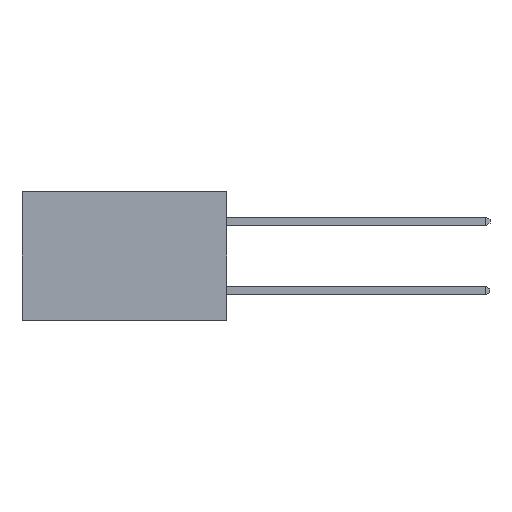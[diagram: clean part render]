
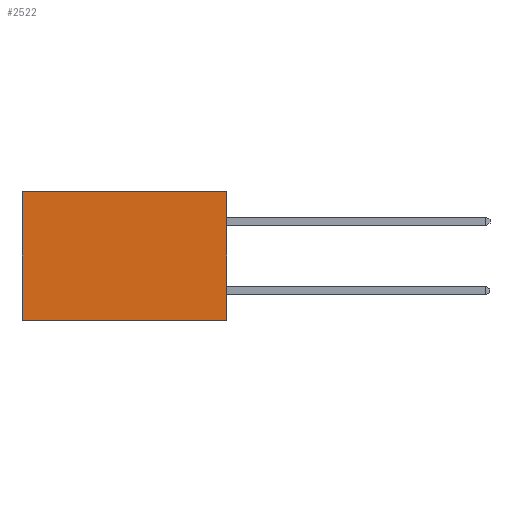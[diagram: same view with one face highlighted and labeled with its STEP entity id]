
A CAD part, left-side view. The second image highlights one B-rep face of the part: STEP entity #2522.
In plain terms, the highlighted planar face has unit normal (-1, 0, 0).
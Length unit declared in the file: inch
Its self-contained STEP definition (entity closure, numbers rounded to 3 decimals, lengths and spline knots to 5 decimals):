
#405 = ORIENTED_EDGE ( 'NONE', *, *, #4401, .F. ) ;
#432 = DIRECTION ( 'NONE',  ( 1., 0., 0. ) ) ;
#1007 = EDGE_LOOP ( 'NONE', ( #6013, #7449, #405, #2501 ) ) ;
#1068 = CARTESIAN_POINT ( 'NONE',  ( 0.277, 0., 0. ) ) ;
#1666 = PLANE ( 'NONE',  #2136 ) ;
#2136 = AXIS2_PLACEMENT_3D ( 'NONE', #5422, #432, #4265 ) ;
#2160 = CARTESIAN_POINT ( 'NONE',  ( 0.277, 0.59, 0. ) ) ;
#2501 = ORIENTED_EDGE ( 'NONE', *, *, #6601, .T. ) ;
#2522 = ADVANCED_FACE ( 'NONE', ( #6278 ), #1666, .F. ) ;
#2627 = CARTESIAN_POINT ( 'NONE',  ( 0.277, 0.59, -0.37 ) ) ;
#2742 = VERTEX_POINT ( 'NONE', #2160 ) ;
#2931 = VERTEX_POINT ( 'NONE', #2627 ) ;
#3594 = LINE ( 'NONE', #4609, #6913 ) ;
#3935 = LINE ( 'NONE', #6629, #7133 ) ;
#4180 = CARTESIAN_POINT ( 'NONE',  ( 0.277, 0., -0.37 ) ) ;
#4265 = DIRECTION ( 'NONE',  ( 0., 0., -1. ) ) ;
#4401 = EDGE_CURVE ( 'NONE', #7000, #7914, #8371, .T. ) ;
#4413 = EDGE_CURVE ( 'NONE', #7914, #2931, #5652, .T. ) ;
#4569 = DIRECTION ( 'NONE',  ( 0., 0., -1. ) ) ;
#4609 = CARTESIAN_POINT ( 'NONE',  ( 0.277, 0.59, -0.37 ) ) ;
#5014 = DIRECTION ( 'NONE',  ( 0., 0., -1. ) ) ;
#5415 = VECTOR ( 'NONE', #7773, 39.37008 ) ;
#5422 = CARTESIAN_POINT ( 'NONE',  ( 0.277, 0., -0.37 ) ) ;
#5652 = LINE ( 'NONE', #7811, #5415 ) ;
#6013 = ORIENTED_EDGE ( 'NONE', *, *, #6222, .T. ) ;
#6222 = EDGE_CURVE ( 'NONE', #2742, #2931, #3594, .T. ) ;
#6278 = FACE_OUTER_BOUND ( 'NONE', #1007, .T. ) ;
#6601 = EDGE_CURVE ( 'NONE', #7000, #2742, #3935, .T. ) ;
#6629 = CARTESIAN_POINT ( 'NONE',  ( 0.277, 0., 0. ) ) ;
#6913 = VECTOR ( 'NONE', #4569, 39.37008 ) ;
#7000 = VERTEX_POINT ( 'NONE', #1068 ) ;
#7029 = VECTOR ( 'NONE', #5014, 39.37008 ) ;
#7119 = DIRECTION ( 'NONE',  ( 0., 1., 0. ) ) ;
#7133 = VECTOR ( 'NONE', #7119, 39.37008 ) ;
#7449 = ORIENTED_EDGE ( 'NONE', *, *, #4413, .F. ) ;
#7773 = DIRECTION ( 'NONE',  ( 0., 1., 0. ) ) ;
#7811 = CARTESIAN_POINT ( 'NONE',  ( 0.277, 0., -0.37 ) ) ;
#7914 = VERTEX_POINT ( 'NONE', #4180 ) ;
#7952 = CARTESIAN_POINT ( 'NONE',  ( 0.277, 0., -0.37 ) ) ;
#8371 = LINE ( 'NONE', #7952, #7029 ) ;
